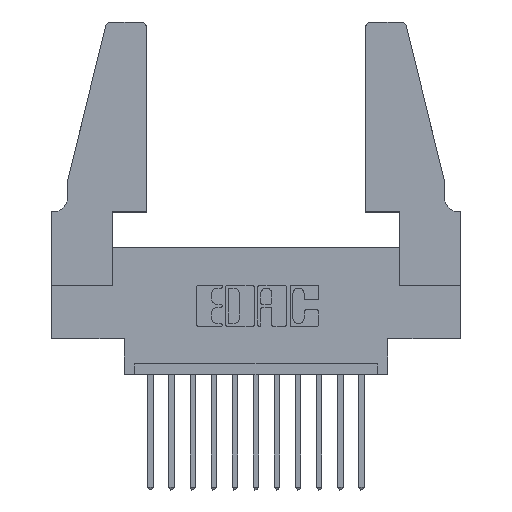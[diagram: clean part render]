
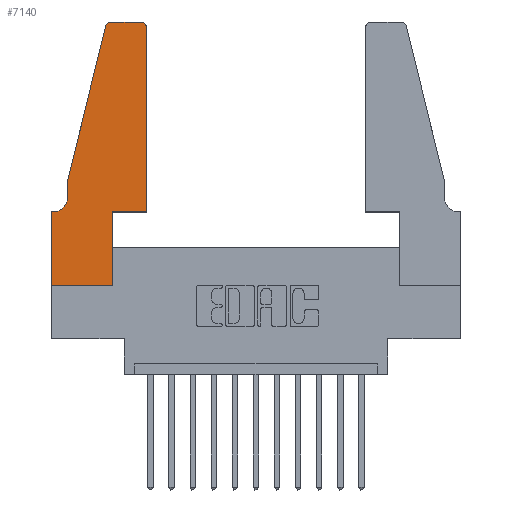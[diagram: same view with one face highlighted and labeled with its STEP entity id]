
A CAD part, top view. The second image highlights one B-rep face of the part: STEP entity #7140.
In plain terms, the highlighted planar face has unit normal (0, 0, 1).
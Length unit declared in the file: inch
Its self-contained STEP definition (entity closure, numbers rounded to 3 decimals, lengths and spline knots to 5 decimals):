
#158 = ORIENTED_EDGE ( 'NONE', *, *, #3544, .T. ) ;
#485 = DIRECTION ( 'NONE',  ( 0., 1., 0. ) ) ;
#621 = VECTOR ( 'NONE', #6634, 39.37008 ) ;
#695 = DIRECTION ( 'NONE',  ( 1., 0., 0. ) ) ;
#777 = FACE_OUTER_BOUND ( 'NONE', #9847, .T. ) ;
#910 = LINE ( 'NONE', #10027, #10741 ) ;
#1123 = VECTOR ( 'NONE', #9990, 39.37008 ) ;
#1199 = ORIENTED_EDGE ( 'NONE', *, *, #13793, .T. ) ;
#1217 = ORIENTED_EDGE ( 'NONE', *, *, #6463, .T. ) ;
#1240 = VECTOR ( 'NONE', #10949, 39.37008 ) ;
#1330 = CARTESIAN_POINT ( 'NONE',  ( 0.25487, 1.22718, 0.37 ) ) ;
#1467 = DIRECTION ( 'NONE',  ( 0., 1., 0. ) ) ;
#1479 = LINE ( 'NONE', #10097, #1123 ) ;
#1489 = VERTEX_POINT ( 'NONE', #14302 ) ;
#1836 = ORIENTED_EDGE ( 'NONE', *, *, #8024, .T. ) ;
#1857 = CARTESIAN_POINT ( 'NONE',  ( 0.4205, 1.22, 0.37 ) ) ;
#2094 = CARTESIAN_POINT ( 'NONE',  ( 0.4505, 0.35, 0.37 ) ) ;
#2125 = LINE ( 'NONE', #7299, #7288 ) ;
#3124 = CIRCLE ( 'NONE', #13273, 0.03 ) ;
#3347 = EDGE_CURVE ( 'NONE', #3484, #6425, #3124, .T. ) ;
#3356 = DIRECTION ( 'NONE',  ( 0., 0., -1. ) ) ;
#3417 = CARTESIAN_POINT ( 'NONE',  ( 0., 0.35, 0.37 ) ) ;
#3484 = VERTEX_POINT ( 'NONE', #11905 ) ;
#3544 = EDGE_CURVE ( 'NONE', #4962, #3484, #1479, .T. ) ;
#3672 = EDGE_CURVE ( 'NONE', #6425, #12737, #7360, .T. ) ;
#3766 = DIRECTION ( 'NONE',  ( 0., -1., 0. ) ) ;
#3780 = LINE ( 'NONE', #6511, #1240 ) ;
#4336 = CIRCLE ( 'NONE', #13864, 0.03 ) ;
#4368 = VECTOR ( 'NONE', #12590, 39.37008 ) ;
#4576 = DIRECTION ( 'NONE',  ( -1., 0., 0. ) ) ;
#4628 = CARTESIAN_POINT ( 'NONE',  ( 0.0755, 0.5, 0.37 ) ) ;
#4763 = DIRECTION ( 'NONE',  ( 1., 0., 0. ) ) ;
#4934 = CARTESIAN_POINT ( 'NONE',  ( 0., 0., 0.37 ) ) ;
#4962 = VERTEX_POINT ( 'NONE', #7331 ) ;
#5033 = DIRECTION ( 'NONE',  ( 0., 0., 1. ) ) ;
#5216 = CARTESIAN_POINT ( 'NONE',  ( 0.4505, 0.35, 0.37 ) ) ;
#5374 = DIRECTION ( 'NONE',  ( 0., -1., 0. ) ) ;
#5443 = EDGE_CURVE ( 'NONE', #6499, #14103, #6785, .T. ) ;
#5763 = CARTESIAN_POINT ( 'NONE',  ( 0.0755, 0.5, 0.37 ) ) ;
#5766 = ORIENTED_EDGE ( 'NONE', *, *, #3672, .T. ) ;
#6175 = CIRCLE ( 'NONE', #9084, 0.07 ) ;
#6425 = VERTEX_POINT ( 'NONE', #1330 ) ;
#6463 = EDGE_CURVE ( 'NONE', #7865, #12236, #14341, .T. ) ;
#6499 = VERTEX_POINT ( 'NONE', #10548 ) ;
#6511 = CARTESIAN_POINT ( 'NONE',  ( 0.0755, 0.35, 0.37 ) ) ;
#6619 = CARTESIAN_POINT ( 'NONE',  ( 0.0055, 0.35, 0.37 ) ) ;
#6634 = DIRECTION ( 'NONE',  ( 1., 0., 0. ) ) ;
#6785 = LINE ( 'NONE', #11959, #8384 ) ;
#7140 = ADVANCED_FACE ( 'NONE', ( #777 ), #10261, .T. ) ;
#7288 = VECTOR ( 'NONE', #1467, 39.37008 ) ;
#7299 = CARTESIAN_POINT ( 'NONE',  ( 0.4505, 0.35, 0.37 ) ) ;
#7331 = CARTESIAN_POINT ( 'NONE',  ( 0.4205, 1.25, 0.37 ) ) ;
#7360 = LINE ( 'NONE', #4628, #4368 ) ;
#7468 = AXIS2_PLACEMENT_3D ( 'NONE', #3417, #9325, #12696 ) ;
#7589 = DIRECTION ( 'NONE',  ( 1., 0., 0. ) ) ;
#7636 = EDGE_CURVE ( 'NONE', #12737, #1489, #10229, .T. ) ;
#7676 = ORIENTED_EDGE ( 'NONE', *, *, #10791, .T. ) ;
#7865 = VERTEX_POINT ( 'NONE', #8512 ) ;
#8024 = EDGE_CURVE ( 'NONE', #12236, #6499, #910, .T. ) ;
#8219 = ORIENTED_EDGE ( 'NONE', *, *, #7636, .T. ) ;
#8384 = VECTOR ( 'NONE', #485, 39.37008 ) ;
#8497 = EDGE_CURVE ( 'NONE', #10666, #7865, #3780, .T. ) ;
#8512 = CARTESIAN_POINT ( 'NONE',  ( 0., 0.35, 0.37 ) ) ;
#9084 = AXIS2_PLACEMENT_3D ( 'NONE', #9262, #3356, #4576 ) ;
#9121 = ORIENTED_EDGE ( 'NONE', *, *, #5443, .T. ) ;
#9262 = CARTESIAN_POINT ( 'NONE',  ( 0.0055, 0.42, 0.37 ) ) ;
#9325 = DIRECTION ( 'NONE',  ( 0., 0., 1. ) ) ;
#9366 = EDGE_CURVE ( 'NONE', #12985, #9994, #2125, .T. ) ;
#9418 = CARTESIAN_POINT ( 'NONE',  ( 0.2865, 0.35, 0.37 ) ) ;
#9784 = CARTESIAN_POINT ( 'NONE',  ( 0.284, 1.22, 0.37 ) ) ;
#9847 = EDGE_LOOP ( 'NONE', ( #158, #11198, #5766, #8219, #7676, #13629, #1217, #1836, #9121, #10263, #12890, #1199 ) ) ;
#9990 = DIRECTION ( 'NONE',  ( -1., 0., 0. ) ) ;
#9994 = VERTEX_POINT ( 'NONE', #10464 ) ;
#10027 = CARTESIAN_POINT ( 'NONE',  ( 0., 0., 0.37 ) ) ;
#10097 = CARTESIAN_POINT ( 'NONE',  ( 0.2605, 1.25, 0.37 ) ) ;
#10229 = LINE ( 'NONE', #11124, #14300 ) ;
#10261 = PLANE ( 'NONE',  #7468 ) ;
#10263 = ORIENTED_EDGE ( 'NONE', *, *, #11337, .T. ) ;
#10464 = CARTESIAN_POINT ( 'NONE',  ( 0.4505, 1.22, 0.37 ) ) ;
#10548 = CARTESIAN_POINT ( 'NONE',  ( 0.2865, 0., 0.37 ) ) ;
#10666 = VERTEX_POINT ( 'NONE', #6619 ) ;
#10741 = VECTOR ( 'NONE', #4763, 39.37008 ) ;
#10791 = EDGE_CURVE ( 'NONE', #1489, #10666, #6175, .T. ) ;
#10949 = DIRECTION ( 'NONE',  ( -1., 0., 0. ) ) ;
#11087 = DIRECTION ( 'NONE',  ( 0., 0., 1. ) ) ;
#11124 = CARTESIAN_POINT ( 'NONE',  ( 0.0755, 0.5, 0.37 ) ) ;
#11198 = ORIENTED_EDGE ( 'NONE', *, *, #3347, .T. ) ;
#11337 = EDGE_CURVE ( 'NONE', #14103, #12985, #13983, .T. ) ;
#11905 = CARTESIAN_POINT ( 'NONE',  ( 0.284, 1.25, 0.37 ) ) ;
#11959 = CARTESIAN_POINT ( 'NONE',  ( 0.2865, 0.35, 0.37 ) ) ;
#12236 = VERTEX_POINT ( 'NONE', #13092 ) ;
#12590 = DIRECTION ( 'NONE',  ( -0.239, -0.971, 0. ) ) ;
#12696 = DIRECTION ( 'NONE',  ( 1., 0., 0. ) ) ;
#12727 = VECTOR ( 'NONE', #3766, 39.37008 ) ;
#12737 = VERTEX_POINT ( 'NONE', #5763 ) ;
#12890 = ORIENTED_EDGE ( 'NONE', *, *, #9366, .T. ) ;
#12985 = VERTEX_POINT ( 'NONE', #5216 ) ;
#13092 = CARTESIAN_POINT ( 'NONE',  ( 0., 0., 0.37 ) ) ;
#13273 = AXIS2_PLACEMENT_3D ( 'NONE', #9784, #5033, #695 ) ;
#13629 = ORIENTED_EDGE ( 'NONE', *, *, #8497, .T. ) ;
#13793 = EDGE_CURVE ( 'NONE', #9994, #4962, #4336, .T. ) ;
#13864 = AXIS2_PLACEMENT_3D ( 'NONE', #1857, #11087, #7589 ) ;
#13983 = LINE ( 'NONE', #2094, #621 ) ;
#14103 = VERTEX_POINT ( 'NONE', #9418 ) ;
#14300 = VECTOR ( 'NONE', #5374, 39.37008 ) ;
#14302 = CARTESIAN_POINT ( 'NONE',  ( 0.0755, 0.42, 0.37 ) ) ;
#14341 = LINE ( 'NONE', #4934, #12727 ) ;
